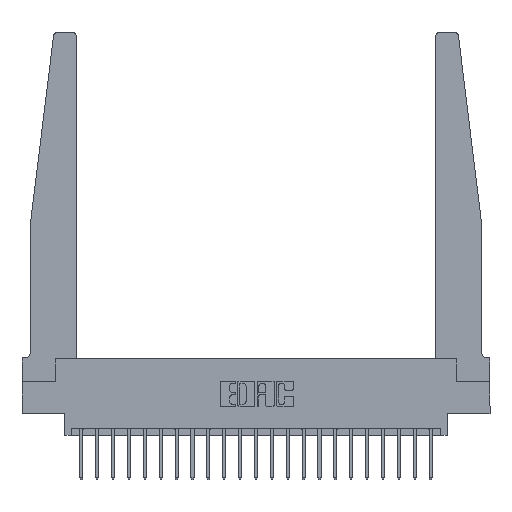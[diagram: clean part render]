
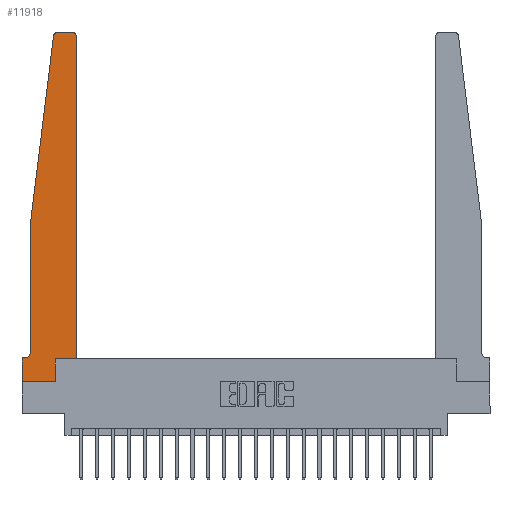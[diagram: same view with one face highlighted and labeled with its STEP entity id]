
A CAD part, top view. The second image highlights one B-rep face of the part: STEP entity #11918.
In plain terms, the highlighted planar face has unit normal (0, 0, 1).
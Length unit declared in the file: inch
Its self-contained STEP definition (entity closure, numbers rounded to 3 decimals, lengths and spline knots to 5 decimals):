
#58 = EDGE_CURVE ( 'NONE', #9350, #7424, #11384, .T. ) ;
#204 = CARTESIAN_POINT ( 'NONE',  ( 0.425, 0.18, 0.37 ) ) ;
#210 = CARTESIAN_POINT ( 'NONE',  ( 0.395, 2.75, 0.37 ) ) ;
#293 = EDGE_CURVE ( 'NONE', #4768, #14365, #12189, .T. ) ;
#560 = DIRECTION ( 'NONE',  ( -0.122, -0.992, 0. ) ) ;
#1799 = CARTESIAN_POINT ( 'NONE',  ( 0.2605, 0.18, 0.37 ) ) ;
#2148 = CARTESIAN_POINT ( 'NONE',  ( 0., 0., 0.37 ) ) ;
#2364 = CARTESIAN_POINT ( 'NONE',  ( 0., 0.1875, 0.37 ) ) ;
#2550 = CARTESIAN_POINT ( 'NONE',  ( 0.27653, 2.72, 0.37 ) ) ;
#2702 = DIRECTION ( 'NONE',  ( 1., 0., 0. ) ) ;
#3272 = EDGE_CURVE ( 'NONE', #15865, #12351, #4855, .T. ) ;
#3554 = ORIENTED_EDGE ( 'NONE', *, *, #21369, .T. ) ;
#3696 = ORIENTED_EDGE ( 'NONE', *, *, #293, .T. ) ;
#3879 = DIRECTION ( 'NONE',  ( 0., 0., 1. ) ) ;
#4233 = VECTOR ( 'NONE', #560, 39.37008 ) ;
#4291 = LINE ( 'NONE', #16368, #18305 ) ;
#4358 = EDGE_CURVE ( 'NONE', #6056, #6571, #13012, .T. ) ;
#4394 = DIRECTION ( 'NONE',  ( 0., 0., -1. ) ) ;
#4512 = CARTESIAN_POINT ( 'NONE',  ( 0., 0., 0.37 ) ) ;
#4520 = DIRECTION ( 'NONE',  ( -1., 0., 0. ) ) ;
#4768 = VERTEX_POINT ( 'NONE', #7409 ) ;
#4855 = LINE ( 'NONE', #6591, #8283 ) ;
#5296 = ORIENTED_EDGE ( 'NONE', *, *, #58, .T. ) ;
#5752 = EDGE_CURVE ( 'NONE', #7424, #11935, #6135, .T. ) ;
#5957 = CARTESIAN_POINT ( 'NONE',  ( 0.425, 0.18, 0.37 ) ) ;
#5993 = VERTEX_POINT ( 'NONE', #204 ) ;
#6056 = VERTEX_POINT ( 'NONE', #7153 ) ;
#6135 = LINE ( 'NONE', #4512, #22839 ) ;
#6411 = CARTESIAN_POINT ( 'NONE',  ( 0.395, 2.72, 0.37 ) ) ;
#6453 = VECTOR ( 'NONE', #20392, 39.37008 ) ;
#6571 = VERTEX_POINT ( 'NONE', #1799 ) ;
#6591 = CARTESIAN_POINT ( 'NONE',  ( 0.25, 2.75, 0.37 ) ) ;
#7153 = CARTESIAN_POINT ( 'NONE',  ( 0.2605, 0., 0.37 ) ) ;
#7180 = CARTESIAN_POINT ( 'NONE',  ( 0.065, 1.25, 0.37 ) ) ;
#7316 = CARTESIAN_POINT ( 'NONE',  ( 0.2605, 0.18, 0.37 ) ) ;
#7409 = CARTESIAN_POINT ( 'NONE',  ( 0.24675, 2.72367, 0.37 ) ) ;
#7424 = VERTEX_POINT ( 'NONE', #20379 ) ;
#7499 = EDGE_CURVE ( 'NONE', #11194, #9350, #18800, .T. ) ;
#7598 = DIRECTION ( 'NONE',  ( 1., 0., 0. ) ) ;
#7930 = DIRECTION ( 'NONE',  ( 0., 0., 1. ) ) ;
#8009 = ORIENTED_EDGE ( 'NONE', *, *, #17400, .T. ) ;
#8067 = AXIS2_PLACEMENT_3D ( 'NONE', #13339, #4394, #22131 ) ;
#8283 = VECTOR ( 'NONE', #17384, 39.37008 ) ;
#9350 = VERTEX_POINT ( 'NONE', #12752 ) ;
#9505 = EDGE_CURVE ( 'NONE', #14365, #11194, #14956, .T. ) ;
#9512 = DIRECTION ( 'NONE',  ( 0., -1., 0. ) ) ;
#9631 = DIRECTION ( 'NONE',  ( 0., 0., 1. ) ) ;
#9864 = CARTESIAN_POINT ( 'NONE',  ( 0.065, 0.2375, 0.37 ) ) ;
#10989 = VERTEX_POINT ( 'NONE', #19047 ) ;
#11093 = PLANE ( 'NONE',  #21388 ) ;
#11130 = CARTESIAN_POINT ( 'NONE',  ( 0.065, 1.25, 0.37 ) ) ;
#11194 = VERTEX_POINT ( 'NONE', #9864 ) ;
#11367 = ORIENTED_EDGE ( 'NONE', *, *, #15417, .T. ) ;
#11371 = DIRECTION ( 'NONE',  ( 0., 1., 0. ) ) ;
#11384 = LINE ( 'NONE', #21923, #16125 ) ;
#11759 = ORIENTED_EDGE ( 'NONE', *, *, #3272, .T. ) ;
#11918 = ADVANCED_FACE ( 'NONE', ( #14702 ), #11093, .T. ) ;
#11935 = VERTEX_POINT ( 'NONE', #2148 ) ;
#12189 = LINE ( 'NONE', #11130, #4233 ) ;
#12351 = VERTEX_POINT ( 'NONE', #19508 ) ;
#12527 = VECTOR ( 'NONE', #15493, 39.37008 ) ;
#12752 = CARTESIAN_POINT ( 'NONE',  ( 0.015, 0.1875, 0.37 ) ) ;
#13012 = LINE ( 'NONE', #7316, #14273 ) ;
#13339 = CARTESIAN_POINT ( 'NONE',  ( 0.015, 0.2375, 0.37 ) ) ;
#14273 = VECTOR ( 'NONE', #20064, 39.37008 ) ;
#14365 = VERTEX_POINT ( 'NONE', #7180 ) ;
#14702 = FACE_OUTER_BOUND ( 'NONE', #17924, .T. ) ;
#14864 = ORIENTED_EDGE ( 'NONE', *, *, #21100, .T. ) ;
#14956 = LINE ( 'NONE', #22135, #12527 ) ;
#15201 = ORIENTED_EDGE ( 'NONE', *, *, #7499, .T. ) ;
#15304 = DIRECTION ( 'NONE',  ( 1., 0., 0. ) ) ;
#15417 = EDGE_CURVE ( 'NONE', #10989, #15865, #18095, .T. ) ;
#15493 = DIRECTION ( 'NONE',  ( 0., -1., 0. ) ) ;
#15701 = ORIENTED_EDGE ( 'NONE', *, *, #9505, .T. ) ;
#15865 = VERTEX_POINT ( 'NONE', #210 ) ;
#15871 = ORIENTED_EDGE ( 'NONE', *, *, #22065, .T. ) ;
#16125 = VECTOR ( 'NONE', #4520, 39.37008 ) ;
#16368 = CARTESIAN_POINT ( 'NONE',  ( 0.425, 0.18, 0.37 ) ) ;
#17036 = CARTESIAN_POINT ( 'NONE',  ( 0., 0., 0.37 ) ) ;
#17384 = DIRECTION ( 'NONE',  ( -1., 0., 0. ) ) ;
#17400 = EDGE_CURVE ( 'NONE', #12351, #4768, #18631, .T. ) ;
#17924 = EDGE_LOOP ( 'NONE', ( #11759, #8009, #3696, #15701, #15201, #5296, #21236, #3554, #21099, #15871, #14864, #11367 ) ) ;
#18095 = CIRCLE ( 'NONE', #21054, 0.03 ) ;
#18305 = VECTOR ( 'NONE', #11371, 39.37008 ) ;
#18631 = CIRCLE ( 'NONE', #21613, 0.03 ) ;
#18800 = CIRCLE ( 'NONE', #8067, 0.05 ) ;
#19047 = CARTESIAN_POINT ( 'NONE',  ( 0.425, 2.72, 0.37 ) ) ;
#19508 = CARTESIAN_POINT ( 'NONE',  ( 0.27653, 2.75, 0.37 ) ) ;
#19648 = LINE ( 'NONE', #5957, #22054 ) ;
#19763 = DIRECTION ( 'NONE',  ( 1., 0., 0. ) ) ;
#20064 = DIRECTION ( 'NONE',  ( 0., 1., 0. ) ) ;
#20379 = CARTESIAN_POINT ( 'NONE',  ( 0., 0.1875, 0.37 ) ) ;
#20392 = DIRECTION ( 'NONE',  ( 1., 0., 0. ) ) ;
#20844 = LINE ( 'NONE', #17036, #6453 ) ;
#21054 = AXIS2_PLACEMENT_3D ( 'NONE', #6411, #7930, #2702 ) ;
#21099 = ORIENTED_EDGE ( 'NONE', *, *, #4358, .T. ) ;
#21100 = EDGE_CURVE ( 'NONE', #5993, #10989, #4291, .T. ) ;
#21236 = ORIENTED_EDGE ( 'NONE', *, *, #5752, .T. ) ;
#21369 = EDGE_CURVE ( 'NONE', #11935, #6056, #20844, .T. ) ;
#21388 = AXIS2_PLACEMENT_3D ( 'NONE', #2364, #3879, #7598 ) ;
#21613 = AXIS2_PLACEMENT_3D ( 'NONE', #2550, #9631, #15304 ) ;
#21923 = CARTESIAN_POINT ( 'NONE',  ( 0.065, 0.1875, 0.37 ) ) ;
#22054 = VECTOR ( 'NONE', #19763, 39.37008 ) ;
#22065 = EDGE_CURVE ( 'NONE', #6571, #5993, #19648, .T. ) ;
#22131 = DIRECTION ( 'NONE',  ( -1., 0., 0. ) ) ;
#22135 = CARTESIAN_POINT ( 'NONE',  ( 0.065, 1.25, 0.37 ) ) ;
#22839 = VECTOR ( 'NONE', #9512, 39.37008 ) ;
